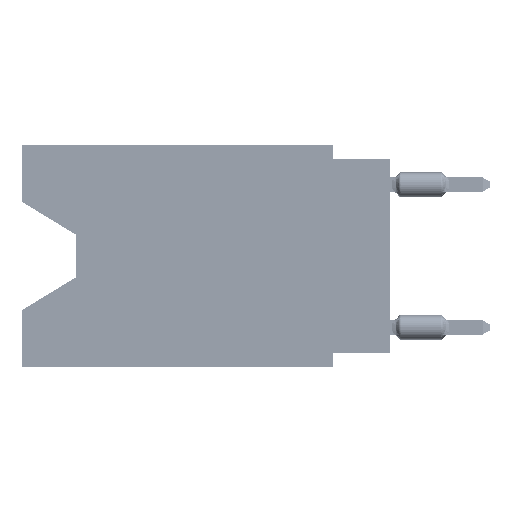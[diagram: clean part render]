
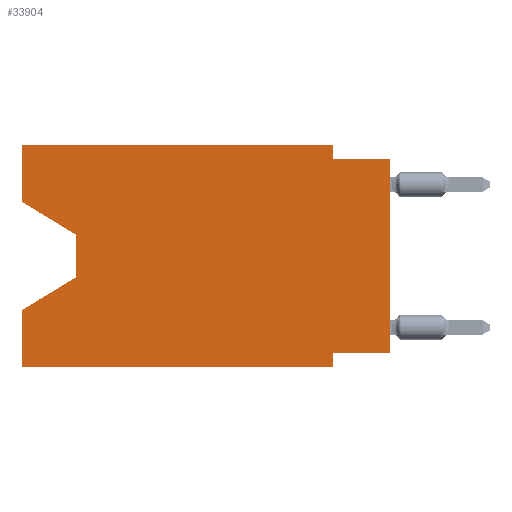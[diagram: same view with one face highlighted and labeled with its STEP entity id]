
A CAD part, left-side view. The second image highlights one B-rep face of the part: STEP entity #33904.
In plain terms, the highlighted planar face has unit normal (-1, 0, 0).
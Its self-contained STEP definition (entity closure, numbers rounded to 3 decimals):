
#1092 = VERTEX_POINT ( 'NONE', #37754 ) ;
#1862 = EDGE_CURVE ( 'NONE', #46370, #1092, #35553, .T. ) ;
#2708 = VERTEX_POINT ( 'NONE', #4970 ) ;
#3652 = LINE ( 'NONE', #72922, #55864 ) ;
#4183 = LINE ( 'NONE', #69191, #25022 ) ;
#4970 = CARTESIAN_POINT ( 'NONE',  ( 0., 2.54, 0. ) ) ;
#5326 = DIRECTION ( 'NONE',  ( 0., 0., 1. ) ) ;
#5408 = EDGE_CURVE ( 'NONE', #12427, #54983, #50696, .T. ) ;
#7398 = CARTESIAN_POINT ( 'NONE',  ( 0., 16.383, -2.546 ) ) ;
#8520 = CARTESIAN_POINT ( 'NONE',  ( 0., 16.383, 0. ) ) ;
#8641 = CARTESIAN_POINT ( 'NONE',  ( 0., 16.383, -9.906 ) ) ;
#8984 = DIRECTION ( 'NONE',  ( 0., 0.855, -0.519 ) ) ;
#9019 = DIRECTION ( 'NONE',  ( 0., -1., 0. ) ) ;
#11451 = VECTOR ( 'NONE', #59941, 1000. ) ;
#12427 = VERTEX_POINT ( 'NONE', #63271 ) ;
#13167 = LINE ( 'NONE', #7398, #59406 ) ;
#13717 = LINE ( 'NONE', #54531, #11451 ) ;
#13954 = VECTOR ( 'NONE', #34980, 1000. ) ;
#14022 = LINE ( 'NONE', #64197, #39948 ) ;
#15819 = EDGE_CURVE ( 'NONE', #26970, #54265, #22292, .T. ) ;
#16445 = VERTEX_POINT ( 'NONE', #19455 ) ;
#17286 = CARTESIAN_POINT ( 'NONE',  ( 0., 16.383, 0. ) ) ;
#17489 = EDGE_CURVE ( 'NONE', #16445, #28198, #14022, .T. ) ;
#19455 = CARTESIAN_POINT ( 'NONE',  ( 0., 16.383, -9.906 ) ) ;
#19695 = LINE ( 'NONE', #47819, #36708 ) ;
#19951 = ORIENTED_EDGE ( 'NONE', *, *, #29868, .T. ) ;
#20152 = ORIENTED_EDGE ( 'NONE', *, *, #15819, .F. ) ;
#20158 = CARTESIAN_POINT ( 'NONE',  ( 0., 13.97, -5.893 ) ) ;
#22292 = LINE ( 'NONE', #69221, #13954 ) ;
#23463 = PLANE ( 'NONE',  #42473 ) ;
#25022 = VECTOR ( 'NONE', #52252, 1000. ) ;
#25873 = DIRECTION ( 'NONE',  ( 0., -1., 0. ) ) ;
#26350 = VECTOR ( 'NONE', #56480, 1000. ) ;
#26970 = VERTEX_POINT ( 'NONE', #70887 ) ;
#27106 = LINE ( 'NONE', #8641, #56971 ) ;
#28198 = VERTEX_POINT ( 'NONE', #57064 ) ;
#29868 = EDGE_CURVE ( 'NONE', #1092, #28198, #72889, .T. ) ;
#30872 = DIRECTION ( 'NONE',  ( 0., -0.855, -0.519 ) ) ;
#31206 = ORIENTED_EDGE ( 'NONE', *, *, #39483, .F. ) ;
#31595 = VERTEX_POINT ( 'NONE', #39305 ) ;
#31633 = LINE ( 'NONE', #55107, #66733 ) ;
#33904 = ADVANCED_FACE ( 'NONE', ( #47307 ), #23463, .F. ) ;
#34980 = DIRECTION ( 'NONE',  ( 0., 0., 1. ) ) ;
#35553 = LINE ( 'NONE', #70553, #57792 ) ;
#36708 = VECTOR ( 'NONE', #72799, 1000. ) ;
#37754 = CARTESIAN_POINT ( 'NONE',  ( 0., 13.97, -5.893 ) ) ;
#38390 = VECTOR ( 'NONE', #8984, 1000. ) ;
#39170 = CARTESIAN_POINT ( 'NONE',  ( 0., 0., -9.271 ) ) ;
#39305 = CARTESIAN_POINT ( 'NONE',  ( 0., 2.54, -9.906 ) ) ;
#39483 = EDGE_CURVE ( 'NONE', #54265, #2708, #19695, .T. ) ;
#39948 = VECTOR ( 'NONE', #5326, 1000. ) ;
#41106 = CARTESIAN_POINT ( 'NONE',  ( 0., 2.54, -9.271 ) ) ;
#42473 = AXIS2_PLACEMENT_3D ( 'NONE', #17286, #70786, #53073 ) ;
#42673 = ORIENTED_EDGE ( 'NONE', *, *, #1862, .T. ) ;
#43061 = ORIENTED_EDGE ( 'NONE', *, *, #63431, .T. ) ;
#45866 = CARTESIAN_POINT ( 'NONE',  ( 0., 13.97, -4.013 ) ) ;
#46233 = ORIENTED_EDGE ( 'NONE', *, *, #73907, .T. ) ;
#46370 = VERTEX_POINT ( 'NONE', #45866 ) ;
#47307 = FACE_OUTER_BOUND ( 'NONE', #53039, .T. ) ;
#47819 = CARTESIAN_POINT ( 'NONE',  ( 0., 16.383, 0. ) ) ;
#47842 = ORIENTED_EDGE ( 'NONE', *, *, #75782, .F. ) ;
#50696 = LINE ( 'NONE', #39170, #26350 ) ;
#52252 = DIRECTION ( 'NONE',  ( 0., 0., 1. ) ) ;
#53039 = EDGE_LOOP ( 'NONE', ( #61897, #42673, #19951, #65793, #43061, #47842, #74066, #46233, #53194, #68387, #31206, #20152 ) ) ;
#53073 = DIRECTION ( 'NONE',  ( 0., 0., -1. ) ) ;
#53188 = VERTEX_POINT ( 'NONE', #69109 ) ;
#53194 = ORIENTED_EDGE ( 'NONE', *, *, #62704, .F. ) ;
#54265 = VERTEX_POINT ( 'NONE', #8520 ) ;
#54531 = CARTESIAN_POINT ( 'NONE',  ( 0., 2.54, 0. ) ) ;
#54983 = VERTEX_POINT ( 'NONE', #41106 ) ;
#55107 = CARTESIAN_POINT ( 'NONE',  ( 0., 0., -0.635 ) ) ;
#55864 = VECTOR ( 'NONE', #66743, 1000. ) ;
#56480 = DIRECTION ( 'NONE',  ( 0., 1., 0. ) ) ;
#56971 = VECTOR ( 'NONE', #9019, 1000. ) ;
#57064 = CARTESIAN_POINT ( 'NONE',  ( 0., 16.383, -7.36 ) ) ;
#57792 = VECTOR ( 'NONE', #59021, 1000. ) ;
#59021 = DIRECTION ( 'NONE',  ( 0., 0., -1. ) ) ;
#59406 = VECTOR ( 'NONE', #30872, 1000. ) ;
#59941 = DIRECTION ( 'NONE',  ( 0., 0., -1. ) ) ;
#61897 = ORIENTED_EDGE ( 'NONE', *, *, #62591, .T. ) ;
#62591 = EDGE_CURVE ( 'NONE', #26970, #46370, #13167, .T. ) ;
#62704 = EDGE_CURVE ( 'NONE', #65462, #53188, #31633, .T. ) ;
#63271 = CARTESIAN_POINT ( 'NONE',  ( 0., 0., -9.271 ) ) ;
#63431 = EDGE_CURVE ( 'NONE', #16445, #31595, #27106, .T. ) ;
#64197 = CARTESIAN_POINT ( 'NONE',  ( 0., 16.383, 0. ) ) ;
#65462 = VERTEX_POINT ( 'NONE', #67614 ) ;
#65793 = ORIENTED_EDGE ( 'NONE', *, *, #17489, .F. ) ;
#66733 = VECTOR ( 'NONE', #25873, 1000. ) ;
#66743 = DIRECTION ( 'NONE',  ( 0., 0., -1. ) ) ;
#67614 = CARTESIAN_POINT ( 'NONE',  ( 0., 2.54, -0.635 ) ) ;
#68387 = ORIENTED_EDGE ( 'NONE', *, *, #72254, .F. ) ;
#69109 = CARTESIAN_POINT ( 'NONE',  ( 0., 0., -0.635 ) ) ;
#69191 = CARTESIAN_POINT ( 'NONE',  ( 0., 0., 0. ) ) ;
#69221 = CARTESIAN_POINT ( 'NONE',  ( 0., 16.383, 0. ) ) ;
#70553 = CARTESIAN_POINT ( 'NONE',  ( 0., 13.97, -4.013 ) ) ;
#70786 = DIRECTION ( 'NONE',  ( 1., 0., 0. ) ) ;
#70887 = CARTESIAN_POINT ( 'NONE',  ( 0., 16.383, -2.546 ) ) ;
#72254 = EDGE_CURVE ( 'NONE', #2708, #65462, #13717, .T. ) ;
#72799 = DIRECTION ( 'NONE',  ( 0., -1., 0. ) ) ;
#72889 = LINE ( 'NONE', #20158, #38390 ) ;
#72922 = CARTESIAN_POINT ( 'NONE',  ( 0., 2.54, -9.906 ) ) ;
#73907 = EDGE_CURVE ( 'NONE', #12427, #53188, #4183, .T. ) ;
#74066 = ORIENTED_EDGE ( 'NONE', *, *, #5408, .F. ) ;
#75782 = EDGE_CURVE ( 'NONE', #54983, #31595, #3652, .T. ) ;
